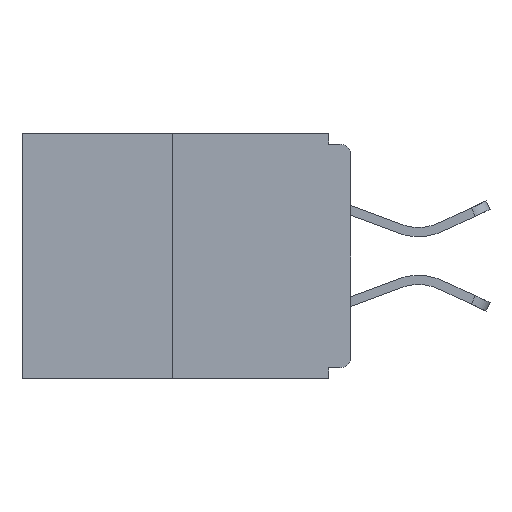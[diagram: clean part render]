
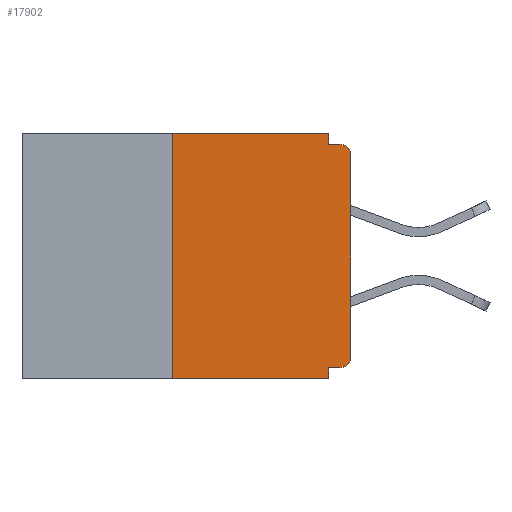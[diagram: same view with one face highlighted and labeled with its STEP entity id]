
A CAD part, left-side view. The second image highlights one B-rep face of the part: STEP entity #17902.
In plain terms, the highlighted planar face has unit normal (-1, 0, 0).
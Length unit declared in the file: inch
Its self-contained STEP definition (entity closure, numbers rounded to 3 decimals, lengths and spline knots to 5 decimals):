
#592 = DIRECTION ( 'NONE',  ( 1., 0., 0. ) ) ;
#961 = CARTESIAN_POINT ( 'NONE',  ( 0., 0., 0. ) ) ;
#1230 = VECTOR ( 'NONE', #20776, 39.37008 ) ;
#1475 = DIRECTION ( 'NONE',  ( 0., 1., 0. ) ) ;
#1755 = VERTEX_POINT ( 'NONE', #11034 ) ;
#1858 = CARTESIAN_POINT ( 'NONE',  ( 0., 0., -0.313 ) ) ;
#1872 = EDGE_CURVE ( 'NONE', #18716, #20051, #4308, .T. ) ;
#2091 = ORIENTED_EDGE ( 'NONE', *, *, #6939, .F. ) ;
#2118 = CARTESIAN_POINT ( 'NONE',  ( 0., 0.25, -0.343 ) ) ;
#2177 = AXIS2_PLACEMENT_3D ( 'NONE', #7119, #592, #13665 ) ;
#2290 = LINE ( 'NONE', #10289, #10896 ) ;
#2583 = CIRCLE ( 'NONE', #13254, 0.015 ) ;
#3231 = CARTESIAN_POINT ( 'NONE',  ( 0., 0.015, -0.328 ) ) ;
#3267 = VECTOR ( 'NONE', #8151, 39.37008 ) ;
#3614 = CARTESIAN_POINT ( 'NONE',  ( 0., 0.46, -0.343 ) ) ;
#4245 = ORIENTED_EDGE ( 'NONE', *, *, #18382, .T. ) ;
#4308 = LINE ( 'NONE', #13026, #10879 ) ;
#4648 = FACE_OUTER_BOUND ( 'NONE', #6328, .T. ) ;
#5182 = CARTESIAN_POINT ( 'NONE',  ( 0., 0.015, -0.015 ) ) ;
#6328 = EDGE_LOOP ( 'NONE', ( #22428, #13184, #4245, #26518, #2091, #9572, #19589, #7162, #12046, #26300 ) ) ;
#6462 = DIRECTION ( 'NONE',  ( 0., 0., -1. ) ) ;
#6939 = EDGE_CURVE ( 'NONE', #22250, #12007, #2290, .T. ) ;
#7119 = CARTESIAN_POINT ( 'NONE',  ( 0., 0.46, 0. ) ) ;
#7162 = ORIENTED_EDGE ( 'NONE', *, *, #17997, .T. ) ;
#7701 = VECTOR ( 'NONE', #26538, 39.37008 ) ;
#8151 = DIRECTION ( 'NONE',  ( 0., -1., 0. ) ) ;
#8673 = CARTESIAN_POINT ( 'NONE',  ( 0., 0.031, -0.343 ) ) ;
#9124 = PLANE ( 'NONE',  #2177 ) ;
#9572 = ORIENTED_EDGE ( 'NONE', *, *, #18337, .T. ) ;
#9927 = VECTOR ( 'NONE', #26511, 39.37008 ) ;
#10289 = CARTESIAN_POINT ( 'NONE',  ( 0., 0., -0.328 ) ) ;
#10879 = VECTOR ( 'NONE', #6462, 39.37008 ) ;
#10896 = VECTOR ( 'NONE', #1475, 39.37008 ) ;
#11034 = CARTESIAN_POINT ( 'NONE',  ( 0., 0.25, 0. ) ) ;
#11053 = CARTESIAN_POINT ( 'NONE',  ( 0., 0.46, 0. ) ) ;
#11077 = DIRECTION ( 'NONE',  ( 0., -1., 0. ) ) ;
#12007 = VERTEX_POINT ( 'NONE', #12909 ) ;
#12046 = ORIENTED_EDGE ( 'NONE', *, *, #18830, .F. ) ;
#12909 = CARTESIAN_POINT ( 'NONE',  ( 0., 0.031, -0.328 ) ) ;
#12927 = LINE ( 'NONE', #961, #1230 ) ;
#13026 = CARTESIAN_POINT ( 'NONE',  ( 0., 0.031, 0. ) ) ;
#13184 = ORIENTED_EDGE ( 'NONE', *, *, #16234, .F. ) ;
#13254 = AXIS2_PLACEMENT_3D ( 'NONE', #14410, #14591, #23292 ) ;
#13665 = DIRECTION ( 'NONE',  ( 0., 0., -1. ) ) ;
#14410 = CARTESIAN_POINT ( 'NONE',  ( 0., 0.015, -0.313 ) ) ;
#14591 = DIRECTION ( 'NONE',  ( -1., 0., 0. ) ) ;
#15126 = CARTESIAN_POINT ( 'NONE',  ( 0., 0.031, -0.015 ) ) ;
#15448 = AXIS2_PLACEMENT_3D ( 'NONE', #23413, #16572, #16763 ) ;
#16113 = EDGE_CURVE ( 'NONE', #1755, #18716, #19945, .T. ) ;
#16234 = EDGE_CURVE ( 'NONE', #23684, #1755, #27255, .T. ) ;
#16346 = LINE ( 'NONE', #8673, #7701 ) ;
#16572 = DIRECTION ( 'NONE',  ( -1., 0., 0. ) ) ;
#16763 = DIRECTION ( 'NONE',  ( 0., 0., -1. ) ) ;
#17461 = CARTESIAN_POINT ( 'NONE',  ( 0., 0., -0.015 ) ) ;
#17902 = ADVANCED_FACE ( 'NONE', ( #4648 ), #9124, .F. ) ;
#17997 = EDGE_CURVE ( 'NONE', #28059, #26761, #27827, .T. ) ;
#18337 = EDGE_CURVE ( 'NONE', #22250, #25345, #2583, .T. ) ;
#18382 = EDGE_CURVE ( 'NONE', #23684, #26943, #24324, .T. ) ;
#18716 = VERTEX_POINT ( 'NONE', #24394 ) ;
#18830 = EDGE_CURVE ( 'NONE', #20051, #26761, #22912, .T. ) ;
#18841 = EDGE_CURVE ( 'NONE', #12007, #26943, #16346, .T. ) ;
#19589 = ORIENTED_EDGE ( 'NONE', *, *, #27821, .T. ) ;
#19945 = LINE ( 'NONE', #11053, #9927 ) ;
#20051 = VERTEX_POINT ( 'NONE', #15126 ) ;
#20477 = CARTESIAN_POINT ( 'NONE',  ( 0., 0.25, 0. ) ) ;
#20776 = DIRECTION ( 'NONE',  ( 0., 0., 1. ) ) ;
#21335 = VECTOR ( 'NONE', #24858, 39.37008 ) ;
#21637 = CARTESIAN_POINT ( 'NONE',  ( 0., 0., -0.03 ) ) ;
#22250 = VERTEX_POINT ( 'NONE', #3231 ) ;
#22428 = ORIENTED_EDGE ( 'NONE', *, *, #16113, .F. ) ;
#22912 = LINE ( 'NONE', #17461, #25322 ) ;
#23292 = DIRECTION ( 'NONE',  ( 0., 0., -1. ) ) ;
#23413 = CARTESIAN_POINT ( 'NONE',  ( 0., 0.015, -0.03 ) ) ;
#23684 = VERTEX_POINT ( 'NONE', #2118 ) ;
#24324 = LINE ( 'NONE', #3614, #3267 ) ;
#24394 = CARTESIAN_POINT ( 'NONE',  ( 0., 0.031, 0. ) ) ;
#24858 = DIRECTION ( 'NONE',  ( 0., 0., 1. ) ) ;
#25322 = VECTOR ( 'NONE', #11077, 39.37008 ) ;
#25345 = VERTEX_POINT ( 'NONE', #1858 ) ;
#25621 = CARTESIAN_POINT ( 'NONE',  ( 0., 0.031, -0.343 ) ) ;
#26300 = ORIENTED_EDGE ( 'NONE', *, *, #1872, .F. ) ;
#26511 = DIRECTION ( 'NONE',  ( 0., -1., 0. ) ) ;
#26518 = ORIENTED_EDGE ( 'NONE', *, *, #18841, .F. ) ;
#26538 = DIRECTION ( 'NONE',  ( 0., 0., -1. ) ) ;
#26761 = VERTEX_POINT ( 'NONE', #5182 ) ;
#26943 = VERTEX_POINT ( 'NONE', #25621 ) ;
#27255 = LINE ( 'NONE', #20477, #21335 ) ;
#27821 = EDGE_CURVE ( 'NONE', #25345, #28059, #12927, .T. ) ;
#27827 = CIRCLE ( 'NONE', #15448, 0.015 ) ;
#28059 = VERTEX_POINT ( 'NONE', #21637 ) ;
